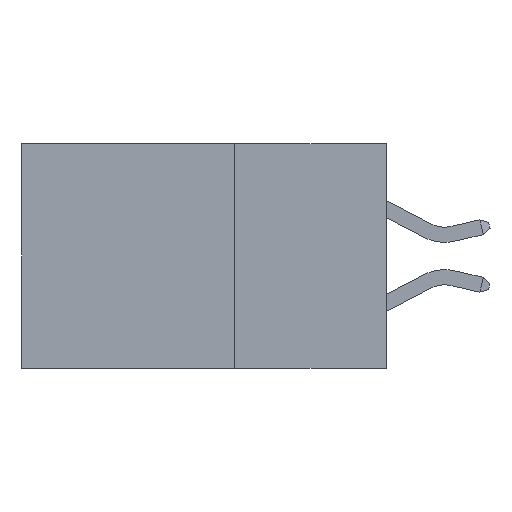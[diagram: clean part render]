
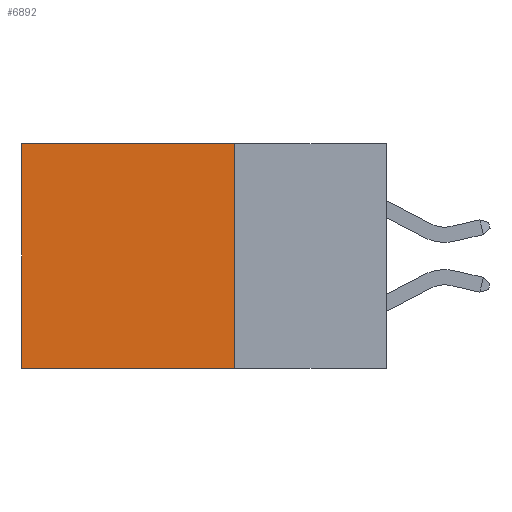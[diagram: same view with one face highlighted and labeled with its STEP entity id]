
A CAD part, left-side view. The second image highlights one B-rep face of the part: STEP entity #6892.
In plain terms, the highlighted planar face has unit normal (-1, 0, 0).
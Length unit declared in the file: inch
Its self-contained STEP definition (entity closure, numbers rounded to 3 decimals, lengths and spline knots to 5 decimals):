
#449 = VECTOR ( 'NONE', #1303, 39.37008 ) ;
#801 = AXIS2_PLACEMENT_3D ( 'NONE', #9915, #12725, #4378 ) ;
#846 = VECTOR ( 'NONE', #11445, 39.37008 ) ;
#925 = CARTESIAN_POINT ( 'NONE',  ( 0.298, 0.6, -0.37 ) ) ;
#1303 = DIRECTION ( 'NONE',  ( 0., 0., -1. ) ) ;
#1580 = PLANE ( 'NONE',  #801 ) ;
#1894 = VERTEX_POINT ( 'NONE', #4105 ) ;
#2200 = EDGE_CURVE ( 'NONE', #1894, #13610, #7427, .T. ) ;
#3141 = VERTEX_POINT ( 'NONE', #17305 ) ;
#3855 = VECTOR ( 'NONE', #12469, 39.37008 ) ;
#4101 = CARTESIAN_POINT ( 'NONE',  ( 0.298, 0.6, 0. ) ) ;
#4105 = CARTESIAN_POINT ( 'NONE',  ( 0.298, 0.25, -0.37 ) ) ;
#4335 = ORIENTED_EDGE ( 'NONE', *, *, #2200, .F. ) ;
#4378 = DIRECTION ( 'NONE',  ( 0., 0., -1. ) ) ;
#5600 = EDGE_LOOP ( 'NONE', ( #11034, #4335, #9781, #8470 ) ) ;
#5861 = CARTESIAN_POINT ( 'NONE',  ( 0.298, 0.25, 0. ) ) ;
#6881 = CARTESIAN_POINT ( 'NONE',  ( 0.298, 0.25, 0. ) ) ;
#6892 = ADVANCED_FACE ( 'NONE', ( #10034 ), #1580, .F. ) ;
#6935 = VERTEX_POINT ( 'NONE', #5861 ) ;
#7302 = EDGE_CURVE ( 'NONE', #6935, #3141, #7611, .T. ) ;
#7427 = LINE ( 'NONE', #15661, #846 ) ;
#7611 = LINE ( 'NONE', #13665, #14493 ) ;
#7612 = LINE ( 'NONE', #4101, #3855 ) ;
#8470 = ORIENTED_EDGE ( 'NONE', *, *, #7302, .T. ) ;
#9781 = ORIENTED_EDGE ( 'NONE', *, *, #15539, .F. ) ;
#9915 = CARTESIAN_POINT ( 'NONE',  ( 0.298, 0.25, 0. ) ) ;
#10034 = FACE_OUTER_BOUND ( 'NONE', #5600, .T. ) ;
#11034 = ORIENTED_EDGE ( 'NONE', *, *, #13279, .T. ) ;
#11445 = DIRECTION ( 'NONE',  ( 0., 1., 0. ) ) ;
#12469 = DIRECTION ( 'NONE',  ( 0., 0., -1. ) ) ;
#12725 = DIRECTION ( 'NONE',  ( 1., 0., 0. ) ) ;
#13279 = EDGE_CURVE ( 'NONE', #3141, #13610, #7612, .T. ) ;
#13610 = VERTEX_POINT ( 'NONE', #925 ) ;
#13665 = CARTESIAN_POINT ( 'NONE',  ( 0.298, 0.25, 0. ) ) ;
#14493 = VECTOR ( 'NONE', #15026, 39.37008 ) ;
#15026 = DIRECTION ( 'NONE',  ( 0., 1., 0. ) ) ;
#15539 = EDGE_CURVE ( 'NONE', #6935, #1894, #15625, .T. ) ;
#15625 = LINE ( 'NONE', #6881, #449 ) ;
#15661 = CARTESIAN_POINT ( 'NONE',  ( 0.298, 0.25, -0.37 ) ) ;
#17305 = CARTESIAN_POINT ( 'NONE',  ( 0.298, 0.6, 0. ) ) ;
